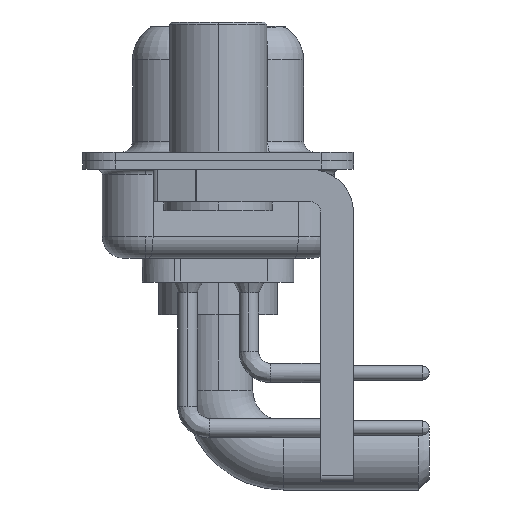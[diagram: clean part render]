
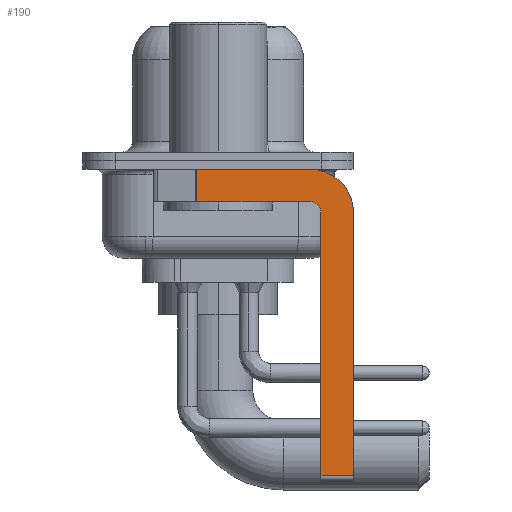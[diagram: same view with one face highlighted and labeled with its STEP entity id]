
A CAD part, left-side view. The second image highlights one B-rep face of the part: STEP entity #190.
In plain terms, the highlighted planar face has unit normal (-1, 0, 0).
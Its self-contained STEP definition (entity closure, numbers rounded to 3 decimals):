
#42 = DIRECTION ( 'NONE',  ( 1., 0., 0. ) ) ;
#121 = VECTOR ( 'NONE', #14538, 1000. ) ;
#190 = ADVANCED_FACE ( 'NONE', ( #15908 ), #5961, .F. ) ;
#468 = EDGE_CURVE ( 'NONE', #14698, #3406, #5094, .T. ) ;
#840 = ORIENTED_EDGE ( 'NONE', *, *, #20447, .F. ) ;
#1001 = CIRCLE ( 'NONE', #3067, 2. ) ;
#1014 = ORIENTED_EDGE ( 'NONE', *, *, #16207, .F. ) ;
#1343 = DIRECTION ( 'NONE',  ( 0., 0., -1. ) ) ;
#1381 = LINE ( 'NONE', #14438, #121 ) ;
#1383 = VERTEX_POINT ( 'NONE', #10574 ) ;
#2500 = VERTEX_POINT ( 'NONE', #18982 ) ;
#2749 = CARTESIAN_POINT ( 'NONE',  ( -2.9, -4.75, -2.4 ) ) ;
#2836 = DIRECTION ( 'NONE',  ( 0., -1., 0. ) ) ;
#2909 = CARTESIAN_POINT ( 'NONE',  ( -2.9, -6.25, -14.55 ) ) ;
#2920 = VECTOR ( 'NONE', #18170, 1000. ) ;
#3067 = AXIS2_PLACEMENT_3D ( 'NONE', #6960, #42, #9714 ) ;
#3406 = VERTEX_POINT ( 'NONE', #2909 ) ;
#4055 = CARTESIAN_POINT ( 'NONE',  ( -2.9, -4.25, -1.9 ) ) ;
#4622 = ORIENTED_EDGE ( 'NONE', *, *, #12871, .F. ) ;
#5094 = LINE ( 'NONE', #11611, #2920 ) ;
#5155 = EDGE_LOOP ( 'NONE', ( #4622, #15130, #1014, #16326, #20227, #18658, #18037, #840 ) ) ;
#5254 = VECTOR ( 'NONE', #2836, 1000. ) ;
#5314 = CARTESIAN_POINT ( 'NONE',  ( -2.9, -4.25, -2.4 ) ) ;
#5326 = VECTOR ( 'NONE', #12160, 1000. ) ;
#5429 = DIRECTION ( 'NONE',  ( 0., -1., 0. ) ) ;
#5961 = PLANE ( 'NONE',  #7703 ) ;
#6177 = CARTESIAN_POINT ( 'NONE',  ( -2.9, -4.25, -2.4 ) ) ;
#6407 = DIRECTION ( 'NONE',  ( 0., 0., -1. ) ) ;
#6769 = VECTOR ( 'NONE', #5429, 1000. ) ;
#6960 = CARTESIAN_POINT ( 'NONE',  ( -2.9, -4.25, -2.4 ) ) ;
#7682 = AXIS2_PLACEMENT_3D ( 'NONE', #5314, #13014, #19782 ) ;
#7703 = AXIS2_PLACEMENT_3D ( 'NONE', #6177, #21053, #1343 ) ;
#8655 = CARTESIAN_POINT ( 'NONE',  ( -2.9, -4.25, -1.9 ) ) ;
#9631 = CARTESIAN_POINT ( 'NONE',  ( -2.9, -4.25, -0.4 ) ) ;
#9714 = DIRECTION ( 'NONE',  ( 0., 0., -1. ) ) ;
#10574 = CARTESIAN_POINT ( 'NONE',  ( -2.9, 0.978, -0.4 ) ) ;
#11016 = LINE ( 'NONE', #11421, #18731 ) ;
#11311 = CARTESIAN_POINT ( 'NONE',  ( -2.9, 0.978, -1.9 ) ) ;
#11421 = CARTESIAN_POINT ( 'NONE',  ( -2.9, 0.978, -1.9 ) ) ;
#11611 = CARTESIAN_POINT ( 'NONE',  ( -2.9, -6.25, -2.4 ) ) ;
#12160 = DIRECTION ( 'NONE',  ( 0., 1., 0. ) ) ;
#12690 = VERTEX_POINT ( 'NONE', #9631 ) ;
#12871 = EDGE_CURVE ( 'NONE', #1383, #12690, #15393, .T. ) ;
#13014 = DIRECTION ( 'NONE',  ( -1., 0., 0. ) ) ;
#13426 = EDGE_CURVE ( 'NONE', #2500, #14406, #1381, .T. ) ;
#13762 = CARTESIAN_POINT ( 'NONE',  ( -2.9, 3., -0.4 ) ) ;
#13997 = EDGE_CURVE ( 'NONE', #14406, #16112, #21031, .T. ) ;
#14406 = VERTEX_POINT ( 'NONE', #2749 ) ;
#14438 = CARTESIAN_POINT ( 'NONE',  ( -2.9, -4.75, -14.8 ) ) ;
#14538 = DIRECTION ( 'NONE',  ( 0., 0., 1. ) ) ;
#14584 = VERTEX_POINT ( 'NONE', #11311 ) ;
#14698 = VERTEX_POINT ( 'NONE', #15263 ) ;
#15130 = ORIENTED_EDGE ( 'NONE', *, *, #18368, .T. ) ;
#15263 = CARTESIAN_POINT ( 'NONE',  ( -2.9, -6.25, -2.4 ) ) ;
#15393 = LINE ( 'NONE', #13762, #5254 ) ;
#15908 = FACE_OUTER_BOUND ( 'NONE', #5155, .T. ) ;
#16112 = VERTEX_POINT ( 'NONE', #8655 ) ;
#16207 = EDGE_CURVE ( 'NONE', #16112, #14584, #18716, .T. ) ;
#16326 = ORIENTED_EDGE ( 'NONE', *, *, #13997, .F. ) ;
#18037 = ORIENTED_EDGE ( 'NONE', *, *, #468, .F. ) ;
#18170 = DIRECTION ( 'NONE',  ( 0., 0., -1. ) ) ;
#18368 = EDGE_CURVE ( 'NONE', #1383, #14584, #11016, .T. ) ;
#18514 = EDGE_CURVE ( 'NONE', #2500, #3406, #19790, .T. ) ;
#18658 = ORIENTED_EDGE ( 'NONE', *, *, #18514, .T. ) ;
#18716 = LINE ( 'NONE', #4055, #5326 ) ;
#18731 = VECTOR ( 'NONE', #6407, 1000. ) ;
#18982 = CARTESIAN_POINT ( 'NONE',  ( -2.9, -4.75, -14.55 ) ) ;
#19782 = DIRECTION ( 'NONE',  ( 0., 0., 1. ) ) ;
#19790 = LINE ( 'NONE', #20112, #6769 ) ;
#20112 = CARTESIAN_POINT ( 'NONE',  ( -2.9, -4.25, -14.55 ) ) ;
#20227 = ORIENTED_EDGE ( 'NONE', *, *, #13426, .F. ) ;
#20447 = EDGE_CURVE ( 'NONE', #12690, #14698, #1001, .T. ) ;
#21031 = CIRCLE ( 'NONE', #7682, 0.5 ) ;
#21053 = DIRECTION ( 'NONE',  ( 1., 0., 0. ) ) ;
